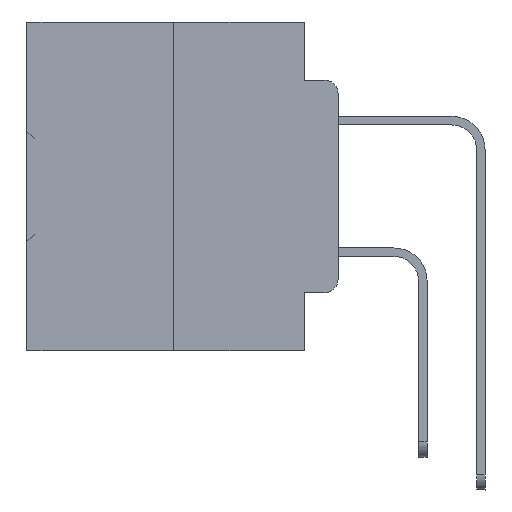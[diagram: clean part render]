
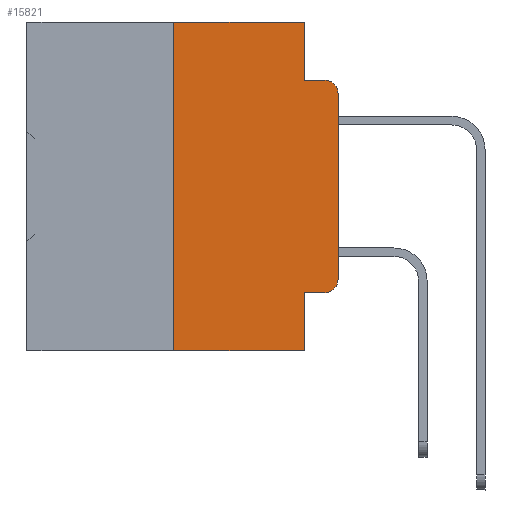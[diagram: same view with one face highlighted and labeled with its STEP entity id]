
A CAD part, left-side view. The second image highlights one B-rep face of the part: STEP entity #15821.
In plain terms, the highlighted planar face has unit normal (-1, 0, 0).
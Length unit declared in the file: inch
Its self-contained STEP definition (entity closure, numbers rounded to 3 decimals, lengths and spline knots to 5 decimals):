
#190 = VECTOR ( 'NONE', #24449, 39.37008 ) ;
#824 = EDGE_CURVE ( 'NONE', #7810, #4178, #7327, .T. ) ;
#843 = CARTESIAN_POINT ( 'NONE',  ( 0., 0.051, -0.5 ) ) ;
#924 = EDGE_CURVE ( 'NONE', #13987, #20109, #30403, .T. ) ;
#1478 = EDGE_CURVE ( 'NONE', #14247, #20109, #20357, .T. ) ;
#1619 = EDGE_CURVE ( 'NONE', #37950, #30743, #8979, .T. ) ;
#1832 = CARTESIAN_POINT ( 'NONE',  ( 0., 0.051, -0.4115 ) ) ;
#1905 = DIRECTION ( 'NONE',  ( 0., 0., -1. ) ) ;
#3026 = ORIENTED_EDGE ( 'NONE', *, *, #824, .T. ) ;
#3209 = CARTESIAN_POINT ( 'NONE',  ( 0., 0.051, 0. ) ) ;
#3619 = DIRECTION ( 'NONE',  ( -1., 0., 0. ) ) ;
#4178 = VERTEX_POINT ( 'NONE', #36511 ) ;
#4895 = CIRCLE ( 'NONE', #16075, 0.02 ) ;
#7327 = LINE ( 'NONE', #19911, #28476 ) ;
#7671 = CARTESIAN_POINT ( 'NONE',  ( 0., 0.051, 0. ) ) ;
#7810 = VERTEX_POINT ( 'NONE', #32719 ) ;
#7992 = VECTOR ( 'NONE', #19645, 39.37008 ) ;
#8953 = ORIENTED_EDGE ( 'NONE', *, *, #37806, .F. ) ;
#8979 = LINE ( 'NONE', #9192, #190 ) ;
#9192 = CARTESIAN_POINT ( 'NONE',  ( 0., 0.473, 0. ) ) ;
#10228 = DIRECTION ( 'NONE',  ( 0., -1., 0. ) ) ;
#10422 = CARTESIAN_POINT ( 'NONE',  ( 0., 0.25, 0. ) ) ;
#10445 = ORIENTED_EDGE ( 'NONE', *, *, #29172, .T. ) ;
#10821 = CARTESIAN_POINT ( 'NONE',  ( 0., 0.25, 0. ) ) ;
#10863 = DIRECTION ( 'NONE',  ( 0., 0., -1. ) ) ;
#11065 = CARTESIAN_POINT ( 'NONE',  ( 0., 0.02, -0.3915 ) ) ;
#11197 = AXIS2_PLACEMENT_3D ( 'NONE', #40265, #36186, #1905 ) ;
#11738 = DIRECTION ( 'NONE',  ( 0., -1., 0. ) ) ;
#12732 = VERTEX_POINT ( 'NONE', #13383 ) ;
#13314 = LINE ( 'NONE', #10422, #33322 ) ;
#13383 = CARTESIAN_POINT ( 'NONE',  ( 0., 0.051, -0.0885 ) ) ;
#13838 = VERTEX_POINT ( 'NONE', #35417 ) ;
#13987 = VERTEX_POINT ( 'NONE', #21331 ) ;
#14247 = VERTEX_POINT ( 'NONE', #18855 ) ;
#14721 = ORIENTED_EDGE ( 'NONE', *, *, #1619, .F. ) ;
#14994 = VERTEX_POINT ( 'NONE', #16222 ) ;
#15821 = ADVANCED_FACE ( 'NONE', ( #30179 ), #18006, .F. ) ;
#15997 = DIRECTION ( 'NONE',  ( 0., 0., 1. ) ) ;
#16075 = AXIS2_PLACEMENT_3D ( 'NONE', #11065, #30453, #10863 ) ;
#16194 = DIRECTION ( 'NONE',  ( 0., 0., -1. ) ) ;
#16222 = CARTESIAN_POINT ( 'NONE',  ( 0., 0.02, -0.0885 ) ) ;
#16612 = LINE ( 'NONE', #26103, #35300 ) ;
#17227 = EDGE_CURVE ( 'NONE', #30743, #12732, #35943, .T. ) ;
#17963 = VECTOR ( 'NONE', #24602, 39.37008 ) ;
#18006 = PLANE ( 'NONE',  #11197 ) ;
#18855 = CARTESIAN_POINT ( 'NONE',  ( 0., 0.051, -0.4115 ) ) ;
#19645 = DIRECTION ( 'NONE',  ( 0., 0., -1. ) ) ;
#19911 = CARTESIAN_POINT ( 'NONE',  ( 0., 0., 0. ) ) ;
#20109 = VERTEX_POINT ( 'NONE', #843 ) ;
#20357 = LINE ( 'NONE', #30045, #35827 ) ;
#21227 = ORIENTED_EDGE ( 'NONE', *, *, #17227, .F. ) ;
#21331 = CARTESIAN_POINT ( 'NONE',  ( 0., 0.25, -0.5 ) ) ;
#23797 = DIRECTION ( 'NONE',  ( 0., 0., 1. ) ) ;
#23932 = ORIENTED_EDGE ( 'NONE', *, *, #36124, .T. ) ;
#23940 = ORIENTED_EDGE ( 'NONE', *, *, #37688, .F. ) ;
#24449 = DIRECTION ( 'NONE',  ( 0., -1., 0. ) ) ;
#24602 = DIRECTION ( 'NONE',  ( 0., -1., 0. ) ) ;
#26103 = CARTESIAN_POINT ( 'NONE',  ( 0., 0.051, -0.0885 ) ) ;
#27945 = ORIENTED_EDGE ( 'NONE', *, *, #924, .T. ) ;
#28371 = EDGE_LOOP ( 'NONE', ( #3026, #32880, #23940, #21227, #14721, #8953, #27945, #38120, #10445, #23932 ) ) ;
#28476 = VECTOR ( 'NONE', #23797, 39.37008 ) ;
#29172 = EDGE_CURVE ( 'NONE', #14247, #13838, #30519, .T. ) ;
#29920 = CIRCLE ( 'NONE', #40450, 0.02 ) ;
#30045 = CARTESIAN_POINT ( 'NONE',  ( 0., 0.051, 0. ) ) ;
#30179 = FACE_OUTER_BOUND ( 'NONE', #28371, .T. ) ;
#30403 = LINE ( 'NONE', #39687, #17963 ) ;
#30453 = DIRECTION ( 'NONE',  ( -1., 0., 0. ) ) ;
#30519 = LINE ( 'NONE', #1832, #36267 ) ;
#30743 = VERTEX_POINT ( 'NONE', #3209 ) ;
#31908 = CARTESIAN_POINT ( 'NONE',  ( 0., 0.02, -0.1085 ) ) ;
#32719 = CARTESIAN_POINT ( 'NONE',  ( 0., 0., -0.3915 ) ) ;
#32880 = ORIENTED_EDGE ( 'NONE', *, *, #36381, .T. ) ;
#33322 = VECTOR ( 'NONE', #15997, 39.37008 ) ;
#35300 = VECTOR ( 'NONE', #10228, 39.37008 ) ;
#35417 = CARTESIAN_POINT ( 'NONE',  ( 0., 0.02, -0.4115 ) ) ;
#35827 = VECTOR ( 'NONE', #36651, 39.37008 ) ;
#35943 = LINE ( 'NONE', #7671, #7992 ) ;
#36124 = EDGE_CURVE ( 'NONE', #13838, #7810, #4895, .T. ) ;
#36186 = DIRECTION ( 'NONE',  ( 1., 0., 0. ) ) ;
#36267 = VECTOR ( 'NONE', #11738, 39.37008 ) ;
#36381 = EDGE_CURVE ( 'NONE', #4178, #14994, #29920, .T. ) ;
#36511 = CARTESIAN_POINT ( 'NONE',  ( 0., 0., -0.1085 ) ) ;
#36651 = DIRECTION ( 'NONE',  ( 0., 0., -1. ) ) ;
#37688 = EDGE_CURVE ( 'NONE', #12732, #14994, #16612, .T. ) ;
#37806 = EDGE_CURVE ( 'NONE', #13987, #37950, #13314, .T. ) ;
#37950 = VERTEX_POINT ( 'NONE', #10821 ) ;
#38120 = ORIENTED_EDGE ( 'NONE', *, *, #1478, .F. ) ;
#39687 = CARTESIAN_POINT ( 'NONE',  ( 0., 0.473, -0.5 ) ) ;
#40265 = CARTESIAN_POINT ( 'NONE',  ( 0., 0.473, 0. ) ) ;
#40450 = AXIS2_PLACEMENT_3D ( 'NONE', #31908, #3619, #16194 ) ;
